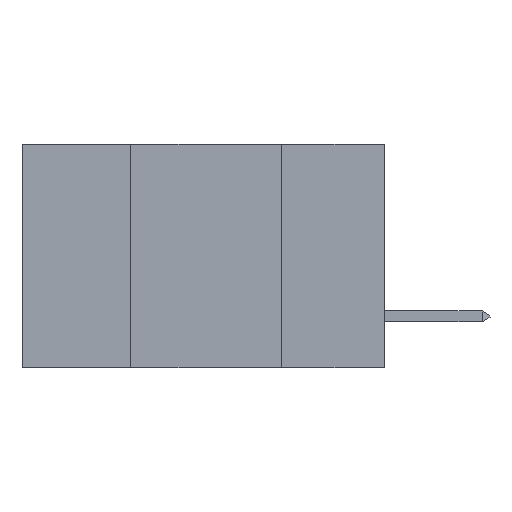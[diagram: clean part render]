
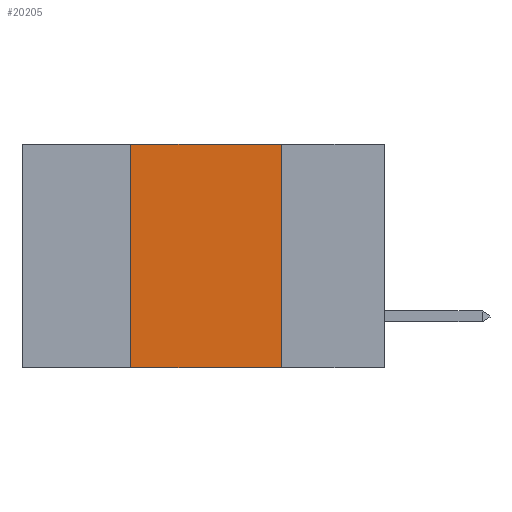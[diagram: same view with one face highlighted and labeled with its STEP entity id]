
A CAD part, left-side view. The second image highlights one B-rep face of the part: STEP entity #20205.
In plain terms, the highlighted planar face has unit normal (-1, 0, 0).
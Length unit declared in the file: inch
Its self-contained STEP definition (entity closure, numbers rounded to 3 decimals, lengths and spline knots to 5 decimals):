
#812 = VECTOR ( 'NONE', #22905, 39.37008 ) ;
#1265 = DIRECTION ( 'NONE',  ( 0., -1., 0. ) ) ;
#1463 = CARTESIAN_POINT ( 'NONE',  ( 0., 0.6, 0. ) ) ;
#2082 = ORIENTED_EDGE ( 'NONE', *, *, #4641, .F. ) ;
#2944 = LINE ( 'NONE', #20511, #10996 ) ;
#3253 = ORIENTED_EDGE ( 'NONE', *, *, #5836, .T. ) ;
#3843 = VERTEX_POINT ( 'NONE', #15380 ) ;
#4074 = VERTEX_POINT ( 'NONE', #10733 ) ;
#4641 = EDGE_CURVE ( 'NONE', #14133, #4074, #17837, .T. ) ;
#4689 = CARTESIAN_POINT ( 'NONE',  ( 0., 0.6, 0. ) ) ;
#5836 = EDGE_CURVE ( 'NONE', #3843, #18998, #2944, .T. ) ;
#6018 = CARTESIAN_POINT ( 'NONE',  ( 0., 0.42, 0. ) ) ;
#6543 = DIRECTION ( 'NONE',  ( 0., 0., -1. ) ) ;
#7087 = EDGE_CURVE ( 'NONE', #3843, #14133, #8967, .T. ) ;
#7731 = DIRECTION ( 'NONE',  ( 0., -1., 0. ) ) ;
#8967 = LINE ( 'NONE', #20302, #22958 ) ;
#10633 = FACE_OUTER_BOUND ( 'NONE', #12050, .T. ) ;
#10733 = CARTESIAN_POINT ( 'NONE',  ( 0., 0.17, 0. ) ) ;
#10996 = VECTOR ( 'NONE', #7731, 39.37008 ) ;
#11989 = EDGE_CURVE ( 'NONE', #4074, #18998, #15406, .T. ) ;
#12050 = EDGE_LOOP ( 'NONE', ( #19240, #2082, #12421, #3253 ) ) ;
#12421 = ORIENTED_EDGE ( 'NONE', *, *, #7087, .F. ) ;
#14133 = VERTEX_POINT ( 'NONE', #6018 ) ;
#15380 = CARTESIAN_POINT ( 'NONE',  ( 0., 0.42, -0.37 ) ) ;
#15406 = LINE ( 'NONE', #19189, #812 ) ;
#17238 = VECTOR ( 'NONE', #1265, 39.37008 ) ;
#17431 = DIRECTION ( 'NONE',  ( 1., 0., 0. ) ) ;
#17440 = CARTESIAN_POINT ( 'NONE',  ( 0., 0.17, -0.37 ) ) ;
#17837 = LINE ( 'NONE', #1463, #17238 ) ;
#18998 = VERTEX_POINT ( 'NONE', #17440 ) ;
#19189 = CARTESIAN_POINT ( 'NONE',  ( 0., 0.17, 0. ) ) ;
#19240 = ORIENTED_EDGE ( 'NONE', *, *, #11989, .F. ) ;
#20205 = ADVANCED_FACE ( 'NONE', ( #10633 ), #21118, .F. ) ;
#20302 = CARTESIAN_POINT ( 'NONE',  ( 0., 0.42, 0. ) ) ;
#20511 = CARTESIAN_POINT ( 'NONE',  ( 0., 0.6, -0.37 ) ) ;
#21118 = PLANE ( 'NONE',  #23715 ) ;
#22139 = DIRECTION ( 'NONE',  ( 0., 0., 1. ) ) ;
#22905 = DIRECTION ( 'NONE',  ( 0., 0., -1. ) ) ;
#22958 = VECTOR ( 'NONE', #22139, 39.37008 ) ;
#23715 = AXIS2_PLACEMENT_3D ( 'NONE', #4689, #17431, #6543 ) ;
